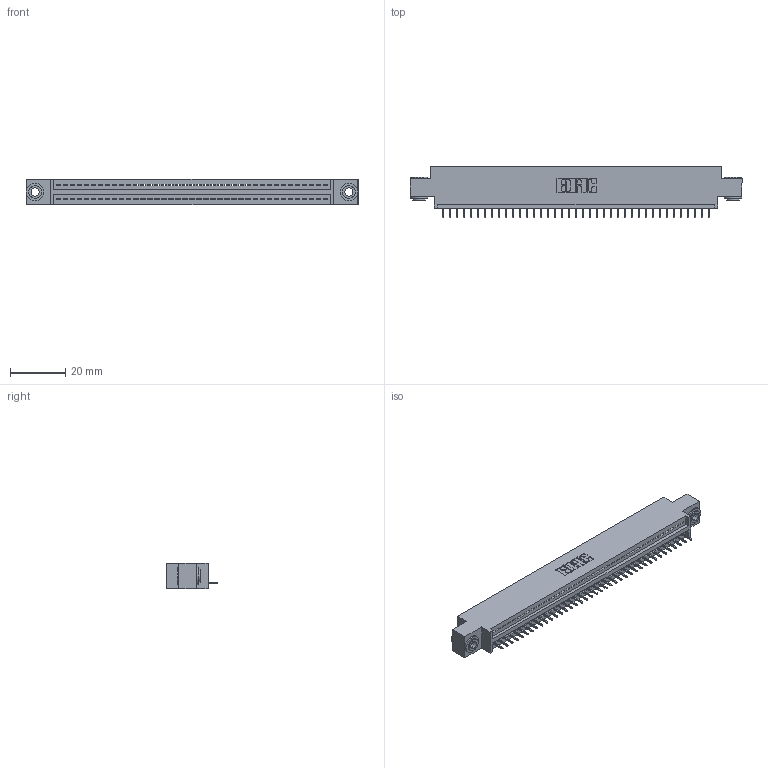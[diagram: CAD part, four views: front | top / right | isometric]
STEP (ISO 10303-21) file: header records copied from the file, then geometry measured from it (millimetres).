
FILE_DESCRIPTION (( 'STEP AP203' ), '1' );
FILE_NAME ('345-039-525-603.STEP', '2020-09-19T18:51:40', ( '' ), ( '' ), 'SwSTEP 2.0', 'SolidWorks 2020', '' );
FILE_SCHEMA (( 'CONFIG_CONTROL_DESIGN' ));
Length unit declared in the file: inch
Products named in the file (4): 345-250-002_345-250-002-102; 345-039-525-603; 345-292-001_345-293-125; 345 Part_0.170 Offset - 0.156 Dia-TH
Assembly tree (42 placements, depth 2):
  345-039-525-603
    345 Part_0.170 Offset - 0.156 Dia-TH
    345-292-001_345-293-125  x39
    345-250-002_345-250-002-102  x2
Bounding box: 120.27 x 18.72 x 9.4 mm (x, y, z)
Volume: 11145.5 mm3; surface area: 14580.6 mm2
Topology: 42 solids, 42 shells, 2586 faces, 7449 edges, 4806 vertices
Faces by surface type: plane 1888, cylinder 690, cone 8
Entity records: 30612 total; most frequent: CARTESIAN_POINT 5280, ORIENTED_EDGE 5246, DIRECTION 4647, EDGE_CURVE 2623, VECTOR 2315, LINE 2315, VERTEX_POINT 1742, AXIS2_PLACEMENT_3D 1166
